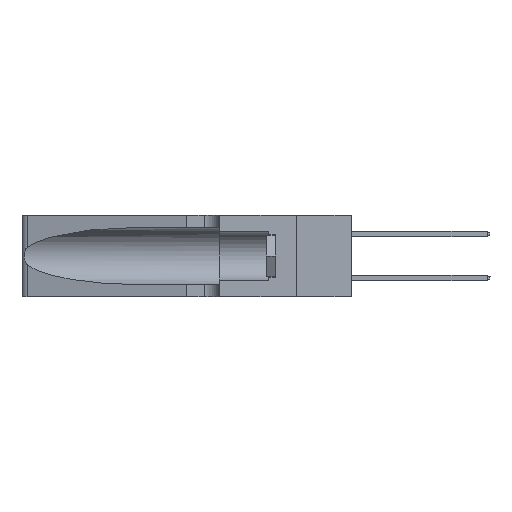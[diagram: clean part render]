
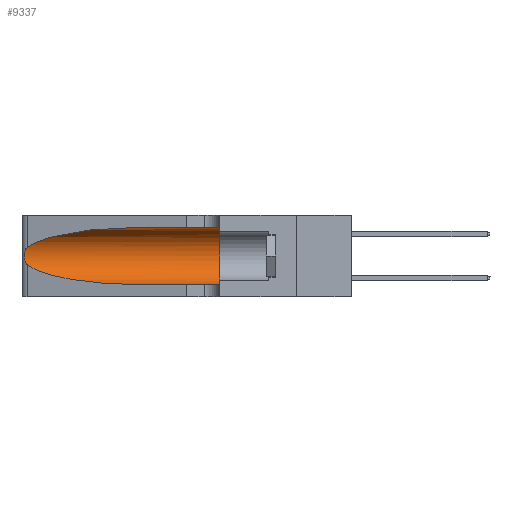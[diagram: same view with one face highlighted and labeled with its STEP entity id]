
A CAD part, left-side view. The second image highlights one B-rep face of the part: STEP entity #9337.
In plain terms, the highlighted cylindrical face has radius 3.308 mm (diameter 6.617 mm), a partial arc.
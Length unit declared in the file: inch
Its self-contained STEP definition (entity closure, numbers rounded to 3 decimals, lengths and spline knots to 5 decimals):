
#591 = CARTESIAN_POINT ( 'NONE',  ( 0.25487, 1.22718, 0.22369 ) ) ;
#602 = AXIS2_PLACEMENT_3D ( 'NONE', #22143, #9110, #24299 ) ;
#823 = CARTESIAN_POINT ( 'NONE',  ( 0.1305, 0.72297, 0.05475 ) ) ;
#892 = CARTESIAN_POINT ( 'NONE',  ( 0.25639, 1.23186, 0.15144 ) ) ;
#2306 = CARTESIAN_POINT ( 'NONE',  ( 0.1305, 1.61858, 0.31525 ) ) ;
#2611 =( BOUNDED_CURVE ( )  B_SPLINE_CURVE ( 3, ( #13580, #22257, #7066, #591 ),
 .UNSPECIFIED., .F., .F. ) 
 B_SPLINE_CURVE_WITH_KNOTS ( ( 4, 4 ),
 ( 1.5708, 2.84003 ),
 .UNSPECIFIED. ) 
 CURVE ( )  GEOMETRIC_REPRESENTATION_ITEM ( )  RATIONAL_B_SPLINE_CURVE ( ( 1., 0.87, 0.87, 1. ) ) 
 REPRESENTATION_ITEM ( '' )  );
#2720 = CARTESIAN_POINT ( 'NONE',  ( 0.1305, 0.35, 0.31525 ) ) ;
#3045 = EDGE_CURVE ( 'NONE', #9475, #25933, #2611, .T. ) ;
#3114 = CARTESIAN_POINT ( 'NONE',  ( 0.25487, 1.22718, 0.14631 ) ) ;
#3987 = CIRCLE ( 'NONE', #602, 0.13025 ) ;
#4480 = DIRECTION ( 'NONE',  ( 0., -1., 0. ) ) ;
#5196 = CARTESIAN_POINT ( 'NONE',  ( 0.25639, 1.23184, 0.21858 ) ) ;
#5541 =( BOUNDED_CURVE ( )  B_SPLINE_CURVE ( 3, ( #26745, #11640, #13820, #823 ),
 .UNSPECIFIED., .F., .F. ) 
 B_SPLINE_CURVE_WITH_KNOTS ( ( 4, 4 ),
 ( 3.44316, 4.71239 ),
 .UNSPECIFIED. ) 
 CURVE ( )  GEOMETRIC_REPRESENTATION_ITEM ( )  RATIONAL_B_SPLINE_CURVE ( ( 1., 0.87, 0.87, 1. ) ) 
 REPRESENTATION_ITEM ( '' )  );
#5982 = VECTOR ( 'NONE', #16078, 39.37008 ) ;
#5988 = CARTESIAN_POINT ( 'NONE',  ( 0.1305, 0.72297, 0.31525 ) ) ;
#7063 = ORIENTED_EDGE ( 'NONE', *, *, #25706, .T. ) ;
#7066 = CARTESIAN_POINT ( 'NONE',  ( 0.2373, 1.15595, 0.28018 ) ) ;
#7356 = CARTESIAN_POINT ( 'NONE',  ( 0.25854, 1.2359, 0.20912 ) ) ;
#7666 = CYLINDRICAL_SURFACE ( 'NONE', #18671, 0.13025 ) ;
#8499 = B_SPLINE_CURVE_WITH_KNOTS ( 'NONE', 3,
 ( #9445, #26726, #5196, #20391, #7356, #22576, #9531, #24717, #11710, #26820, #13888, #892, #16097, #3114 ),
 .UNSPECIFIED., .F., .F.,
 ( 4, 2, 2, 2, 2, 2, 4 ),
 ( 0., 0.00027, 0.00053, 0.00107, 0.0016, 0.00187, 0.00214 ),
 .UNSPECIFIED. ) ;
#9110 = DIRECTION ( 'NONE',  ( 0., 1., 0. ) ) ;
#9337 = ADVANCED_FACE ( 'NONE', ( #19939 ), #7666, .F. ) ;
#9445 = CARTESIAN_POINT ( 'NONE',  ( 0.25487, 1.22718, 0.22369 ) ) ;
#9475 = VERTEX_POINT ( 'NONE', #5988 ) ;
#9531 = CARTESIAN_POINT ( 'NONE',  ( 0.26075, 1.23896, 0.19203 ) ) ;
#9611 = CARTESIAN_POINT ( 'NONE',  ( 0.1305, 1.61858, 0.05475 ) ) ;
#11640 = CARTESIAN_POINT ( 'NONE',  ( 0.2373, 1.15595, 0.08982 ) ) ;
#11710 = CARTESIAN_POINT ( 'NONE',  ( 0.26017, 1.23833, 0.17102 ) ) ;
#11733 = LINE ( 'NONE', #9611, #5982 ) ;
#11772 = ORIENTED_EDGE ( 'NONE', *, *, #12521, .T. ) ;
#12279 = CARTESIAN_POINT ( 'NONE',  ( 0.1305, 0.72297, 0.05475 ) ) ;
#12336 = EDGE_CURVE ( 'NONE', #9475, #27404, #23867, .T. ) ;
#12521 = EDGE_CURVE ( 'NONE', #16832, #23536, #5541, .T. ) ;
#12949 = VECTOR ( 'NONE', #4480, 39.37008 ) ;
#13580 = CARTESIAN_POINT ( 'NONE',  ( 0.1305, 0.72297, 0.31525 ) ) ;
#13820 = CARTESIAN_POINT ( 'NONE',  ( 0.18966, 0.96281, 0.05475 ) ) ;
#13888 = CARTESIAN_POINT ( 'NONE',  ( 0.25789, 1.23486, 0.15765 ) ) ;
#13974 = VERTEX_POINT ( 'NONE', #18418 ) ;
#14138 = DIRECTION ( 'NONE',  ( 0., -1., 0. ) ) ;
#16078 = DIRECTION ( 'NONE',  ( 0., -1., 0. ) ) ;
#16097 = CARTESIAN_POINT ( 'NONE',  ( 0.25555, 1.22993, 0.14849 ) ) ;
#16832 = VERTEX_POINT ( 'NONE', #21287 ) ;
#17034 = ORIENTED_EDGE ( 'NONE', *, *, #12336, .F. ) ;
#17058 = EDGE_CURVE ( 'NONE', #27404, #13974, #3987, .T. ) ;
#18060 = EDGE_LOOP ( 'NONE', ( #20272, #7063, #11772, #19426, #23844, #17034 ) ) ;
#18418 = CARTESIAN_POINT ( 'NONE',  ( 0.1305, 0.35, 0.05475 ) ) ;
#18671 = AXIS2_PLACEMENT_3D ( 'NONE', #24949, #14138, #22816 ) ;
#19426 = ORIENTED_EDGE ( 'NONE', *, *, #26260, .T. ) ;
#19939 = FACE_OUTER_BOUND ( 'NONE', #18060, .T. ) ;
#20272 = ORIENTED_EDGE ( 'NONE', *, *, #3045, .T. ) ;
#20391 = CARTESIAN_POINT ( 'NONE',  ( 0.25787, 1.23484, 0.2124 ) ) ;
#21287 = CARTESIAN_POINT ( 'NONE',  ( 0.25487, 1.22718, 0.14631 ) ) ;
#22143 = CARTESIAN_POINT ( 'NONE',  ( 0.1305, 0.35, 0.185 ) ) ;
#22257 = CARTESIAN_POINT ( 'NONE',  ( 0.18966, 0.96281, 0.31525 ) ) ;
#22576 = CARTESIAN_POINT ( 'NONE',  ( 0.26018, 1.23835, 0.19895 ) ) ;
#22816 = DIRECTION ( 'NONE',  ( 0., 0., -1. ) ) ;
#23536 = VERTEX_POINT ( 'NONE', #12279 ) ;
#23844 = ORIENTED_EDGE ( 'NONE', *, *, #17058, .F. ) ;
#23867 = LINE ( 'NONE', #2306, #12949 ) ;
#24299 = DIRECTION ( 'NONE',  ( 0., 0., 1. ) ) ;
#24717 = CARTESIAN_POINT ( 'NONE',  ( 0.26075, 1.23896, 0.178 ) ) ;
#24949 = CARTESIAN_POINT ( 'NONE',  ( 0.1305, 1.61858, 0.185 ) ) ;
#25440 = CARTESIAN_POINT ( 'NONE',  ( 0.25487, 1.22718, 0.22369 ) ) ;
#25706 = EDGE_CURVE ( 'NONE', #25933, #16832, #8499, .T. ) ;
#25933 = VERTEX_POINT ( 'NONE', #25440 ) ;
#26260 = EDGE_CURVE ( 'NONE', #23536, #13974, #11733, .T. ) ;
#26726 = CARTESIAN_POINT ( 'NONE',  ( 0.25555, 1.22994, 0.2215 ) ) ;
#26745 = CARTESIAN_POINT ( 'NONE',  ( 0.25487, 1.22718, 0.14631 ) ) ;
#26820 = CARTESIAN_POINT ( 'NONE',  ( 0.25856, 1.23593, 0.16098 ) ) ;
#27404 = VERTEX_POINT ( 'NONE', #2720 ) ;
